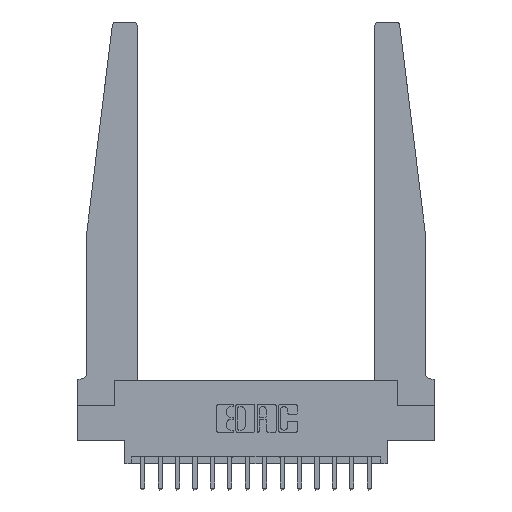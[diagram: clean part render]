
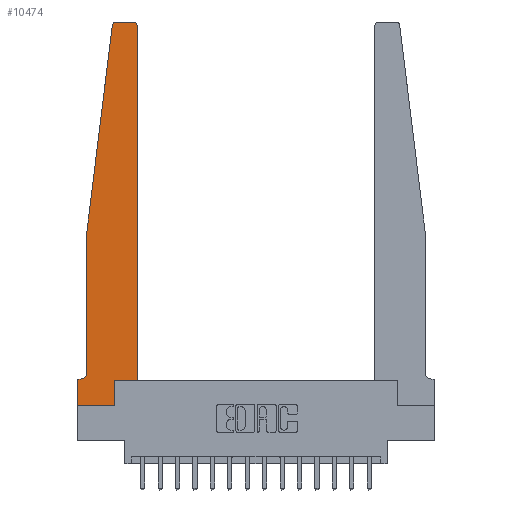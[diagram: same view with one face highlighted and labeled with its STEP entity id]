
A CAD part, top view. The second image highlights one B-rep face of the part: STEP entity #10474.
In plain terms, the highlighted planar face has unit normal (0, 0, 1).
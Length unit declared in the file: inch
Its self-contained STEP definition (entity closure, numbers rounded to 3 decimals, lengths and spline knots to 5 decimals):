
#238 = VERTEX_POINT ( 'NONE', #6701 ) ;
#348 = EDGE_CURVE ( 'NONE', #4270, #4635, #6534, .T. ) ;
#463 = ORIENTED_EDGE ( 'NONE', *, *, #348, .T. ) ;
#977 = VERTEX_POINT ( 'NONE', #3558 ) ;
#1071 = CARTESIAN_POINT ( 'NONE',  ( 0.425, 0.18, 0.37 ) ) ;
#1089 = VECTOR ( 'NONE', #17148, 39.37008 ) ;
#1329 = DIRECTION ( 'NONE',  ( 1., 0., 0. ) ) ;
#2286 = CARTESIAN_POINT ( 'NONE',  ( 0., 0.1875, 0.37 ) ) ;
#2376 = VECTOR ( 'NONE', #2522, 39.37008 ) ;
#2396 = VECTOR ( 'NONE', #12958, 39.37008 ) ;
#2522 = DIRECTION ( 'NONE',  ( 1., 0., 0. ) ) ;
#3181 = ORIENTED_EDGE ( 'NONE', *, *, #15717, .T. ) ;
#3188 = DIRECTION ( 'NONE',  ( -1., 0., 0. ) ) ;
#3246 = ORIENTED_EDGE ( 'NONE', *, *, #6747, .T. ) ;
#3512 = CARTESIAN_POINT ( 'NONE',  ( 0.2605, 0.18, 0.37 ) ) ;
#3558 = CARTESIAN_POINT ( 'NONE',  ( 0.425, 0.18, 0.37 ) ) ;
#3739 = CARTESIAN_POINT ( 'NONE',  ( 0., 0., 0.37 ) ) ;
#3969 = EDGE_CURVE ( 'NONE', #8190, #4270, #13923, .T. ) ;
#4082 = VERTEX_POINT ( 'NONE', #17197 ) ;
#4119 = CARTESIAN_POINT ( 'NONE',  ( 0.015, 0.1875, 0.37 ) ) ;
#4172 = ORIENTED_EDGE ( 'NONE', *, *, #17932, .T. ) ;
#4270 = VERTEX_POINT ( 'NONE', #10820 ) ;
#4432 = ORIENTED_EDGE ( 'NONE', *, *, #10694, .T. ) ;
#4507 = VERTEX_POINT ( 'NONE', #16771 ) ;
#4601 = ORIENTED_EDGE ( 'NONE', *, *, #15909, .T. ) ;
#4635 = VERTEX_POINT ( 'NONE', #10315 ) ;
#4707 = VERTEX_POINT ( 'NONE', #2286 ) ;
#4890 = LINE ( 'NONE', #6237, #1089 ) ;
#5391 = EDGE_CURVE ( 'NONE', #10278, #17217, #8262, .T. ) ;
#5560 = ORIENTED_EDGE ( 'NONE', *, *, #13265, .T. ) ;
#5971 = LINE ( 'NONE', #14723, #16461 ) ;
#6237 = CARTESIAN_POINT ( 'NONE',  ( 0.065, 1.25, 0.37 ) ) ;
#6534 = LINE ( 'NONE', #3512, #13414 ) ;
#6663 = VERTEX_POINT ( 'NONE', #15912 ) ;
#6698 = CARTESIAN_POINT ( 'NONE',  ( 0.24675, 2.72367, 0.37 ) ) ;
#6701 = CARTESIAN_POINT ( 'NONE',  ( 0.425, 2.72, 0.37 ) ) ;
#6747 = EDGE_CURVE ( 'NONE', #17217, #4707, #14912, .T. ) ;
#6916 = CARTESIAN_POINT ( 'NONE',  ( 0.425, 0.18, 0.37 ) ) ;
#7068 = AXIS2_PLACEMENT_3D ( 'NONE', #15359, #7169, #16713 ) ;
#7169 = DIRECTION ( 'NONE',  ( 0., 0., 1. ) ) ;
#7440 = ORIENTED_EDGE ( 'NONE', *, *, #15146, .T. ) ;
#7468 = DIRECTION ( 'NONE',  ( 0., 0., 1. ) ) ;
#7799 = VERTEX_POINT ( 'NONE', #6698 ) ;
#8190 = VERTEX_POINT ( 'NONE', #10098 ) ;
#8201 = CARTESIAN_POINT ( 'NONE',  ( 0.015, 0.2375, 0.37 ) ) ;
#8244 = DIRECTION ( 'NONE',  ( 0., 1., 0. ) ) ;
#8262 = CIRCLE ( 'NONE', #11939, 0.05 ) ;
#8300 = FACE_OUTER_BOUND ( 'NONE', #9895, .T. ) ;
#8399 = CIRCLE ( 'NONE', #12145, 0.03 ) ;
#9573 = DIRECTION ( 'NONE',  ( -1., 0., 0. ) ) ;
#9732 = DIRECTION ( 'NONE',  ( 0., 0., 1. ) ) ;
#9895 = EDGE_LOOP ( 'NONE', ( #7440, #5560, #4432, #3181, #17145, #3246, #4601, #13854, #463, #4172, #16793, #14052 ) ) ;
#10098 = CARTESIAN_POINT ( 'NONE',  ( 0., 0., 0.37 ) ) ;
#10186 = CARTESIAN_POINT ( 'NONE',  ( 0.25, 2.75, 0.37 ) ) ;
#10278 = VERTEX_POINT ( 'NONE', #17928 ) ;
#10308 = VECTOR ( 'NONE', #3188, 39.37008 ) ;
#10315 = CARTESIAN_POINT ( 'NONE',  ( 0.2605, 0.18, 0.37 ) ) ;
#10474 = ADVANCED_FACE ( 'NONE', ( #8300 ), #14295, .T. ) ;
#10541 = DIRECTION ( 'NONE',  ( -0.122, -0.992, 0. ) ) ;
#10694 = EDGE_CURVE ( 'NONE', #7799, #6663, #5971, .T. ) ;
#10820 = CARTESIAN_POINT ( 'NONE',  ( 0.2605, 0., 0.37 ) ) ;
#11233 = VECTOR ( 'NONE', #13454, 39.37008 ) ;
#11939 = AXIS2_PLACEMENT_3D ( 'NONE', #8201, #17732, #9573 ) ;
#12008 = DIRECTION ( 'NONE',  ( 0., 1., 0. ) ) ;
#12145 = AXIS2_PLACEMENT_3D ( 'NONE', #17892, #9732, #1329 ) ;
#12164 = LINE ( 'NONE', #6916, #15759 ) ;
#12616 = EDGE_CURVE ( 'NONE', #977, #238, #12164, .T. ) ;
#12761 = CIRCLE ( 'NONE', #7068, 0.03 ) ;
#12958 = DIRECTION ( 'NONE',  ( 1., 0., 0. ) ) ;
#13265 = EDGE_CURVE ( 'NONE', #4507, #7799, #12761, .T. ) ;
#13356 = LINE ( 'NONE', #3739, #16495 ) ;
#13390 = CARTESIAN_POINT ( 'NONE',  ( 0.065, 0.1875, 0.37 ) ) ;
#13414 = VECTOR ( 'NONE', #12008, 39.37008 ) ;
#13454 = DIRECTION ( 'NONE',  ( -1., 0., 0. ) ) ;
#13496 = LINE ( 'NONE', #1071, #2376 ) ;
#13533 = DIRECTION ( 'NONE',  ( 0., -1., 0. ) ) ;
#13854 = ORIENTED_EDGE ( 'NONE', *, *, #3969, .T. ) ;
#13923 = LINE ( 'NONE', #17024, #2396 ) ;
#14052 = ORIENTED_EDGE ( 'NONE', *, *, #14529, .T. ) ;
#14295 = PLANE ( 'NONE',  #17418 ) ;
#14529 = EDGE_CURVE ( 'NONE', #238, #4082, #8399, .T. ) ;
#14723 = CARTESIAN_POINT ( 'NONE',  ( 0.065, 1.25, 0.37 ) ) ;
#14912 = LINE ( 'NONE', #13390, #11233 ) ;
#15146 = EDGE_CURVE ( 'NONE', #4082, #4507, #17564, .T. ) ;
#15359 = CARTESIAN_POINT ( 'NONE',  ( 0.27653, 2.72, 0.37 ) ) ;
#15641 = CARTESIAN_POINT ( 'NONE',  ( 0., 0.1875, 0.37 ) ) ;
#15717 = EDGE_CURVE ( 'NONE', #6663, #10278, #4890, .T. ) ;
#15759 = VECTOR ( 'NONE', #8244, 39.37008 ) ;
#15909 = EDGE_CURVE ( 'NONE', #4707, #8190, #13356, .T. ) ;
#15912 = CARTESIAN_POINT ( 'NONE',  ( 0.065, 1.25, 0.37 ) ) ;
#16461 = VECTOR ( 'NONE', #10541, 39.37008 ) ;
#16495 = VECTOR ( 'NONE', #13533, 39.37008 ) ;
#16713 = DIRECTION ( 'NONE',  ( 1., 0., 0. ) ) ;
#16771 = CARTESIAN_POINT ( 'NONE',  ( 0.27653, 2.75, 0.37 ) ) ;
#16793 = ORIENTED_EDGE ( 'NONE', *, *, #12616, .T. ) ;
#16985 = DIRECTION ( 'NONE',  ( 1., 0., 0. ) ) ;
#17024 = CARTESIAN_POINT ( 'NONE',  ( 0., 0., 0.37 ) ) ;
#17145 = ORIENTED_EDGE ( 'NONE', *, *, #5391, .T. ) ;
#17148 = DIRECTION ( 'NONE',  ( 0., -1., 0. ) ) ;
#17197 = CARTESIAN_POINT ( 'NONE',  ( 0.395, 2.75, 0.37 ) ) ;
#17217 = VERTEX_POINT ( 'NONE', #4119 ) ;
#17418 = AXIS2_PLACEMENT_3D ( 'NONE', #15641, #7468, #16985 ) ;
#17564 = LINE ( 'NONE', #10186, #10308 ) ;
#17732 = DIRECTION ( 'NONE',  ( 0., 0., -1. ) ) ;
#17892 = CARTESIAN_POINT ( 'NONE',  ( 0.395, 2.72, 0.37 ) ) ;
#17928 = CARTESIAN_POINT ( 'NONE',  ( 0.065, 0.2375, 0.37 ) ) ;
#17932 = EDGE_CURVE ( 'NONE', #4635, #977, #13496, .T. ) ;
